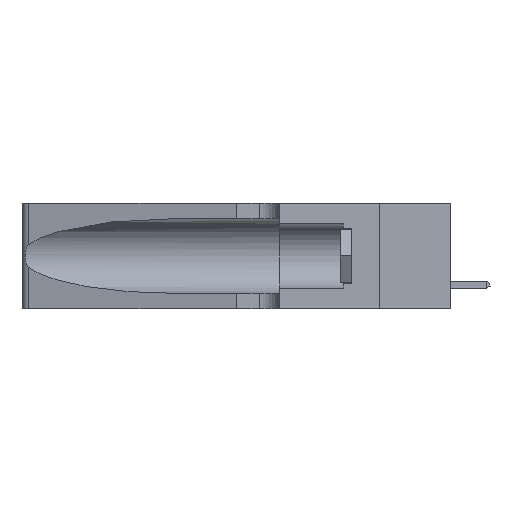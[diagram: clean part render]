
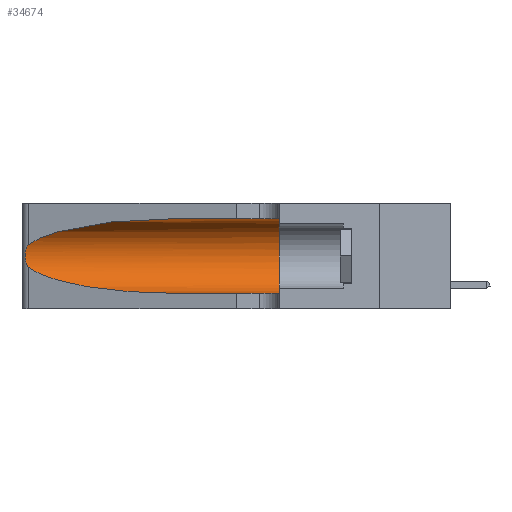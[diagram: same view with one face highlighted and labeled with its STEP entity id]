
A CAD part, left-side view. The second image highlights one B-rep face of the part: STEP entity #34674.
In plain terms, the highlighted cylindrical face has radius 3.308 mm (diameter 6.617 mm), a partial arc.
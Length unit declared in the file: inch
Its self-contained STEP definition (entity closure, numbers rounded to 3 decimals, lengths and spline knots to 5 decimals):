
#932 = EDGE_CURVE ( 'NONE', #12537, #33433, #32184, .T. ) ;
#1087 = VERTEX_POINT ( 'NONE', #41154 ) ;
#1741 = VECTOR ( 'NONE', #4543, 39.37008 ) ;
#1807 = CARTESIAN_POINT ( 'NONE',  ( 0.26018, 1.23835, 0.19895 ) ) ;
#2608 = DIRECTION ( 'NONE',  ( 0., 0., -1. ) ) ;
#2760 = CARTESIAN_POINT ( 'NONE',  ( 0.25487, 1.22718, 0.14631 ) ) ;
#2971 =( BOUNDED_CURVE ( )  B_SPLINE_CURVE ( 3, ( #9185, #18853, #9053, #19129 ),
 .UNSPECIFIED., .F., .T. ) 
 B_SPLINE_CURVE_WITH_KNOTS ( ( 4, 4 ),
 ( 1.5708, 2.84003 ),
 .UNSPECIFIED. ) 
 CURVE ( )  GEOMETRIC_REPRESENTATION_ITEM ( )  RATIONAL_B_SPLINE_CURVE ( ( 1., 0.87, 0.87, 1. ) ) 
 REPRESENTATION_ITEM ( '' )  );
#3777 = LINE ( 'NONE', #27806, #1741 ) ;
#3800 = CARTESIAN_POINT ( 'NONE',  ( 0.25487, 1.22718, 0.22369 ) ) ;
#3946 = FACE_OUTER_BOUND ( 'NONE', #23119, .T. ) ;
#4543 = DIRECTION ( 'NONE',  ( 0., -1., 0. ) ) ;
#4575 = DIRECTION ( 'NONE',  ( 0., 0., 1. ) ) ;
#5106 = CARTESIAN_POINT ( 'NONE',  ( 0.25789, 1.23486, 0.15765 ) ) ;
#8477 =( BOUNDED_CURVE ( )  B_SPLINE_CURVE ( 3, ( #30355, #37179, #30928, #40500 ),
 .UNSPECIFIED., .F., .F. ) 
 B_SPLINE_CURVE_WITH_KNOTS ( ( 4, 4 ),
 ( 3.44316, 4.71239 ),
 .UNSPECIFIED. ) 
 CURVE ( )  GEOMETRIC_REPRESENTATION_ITEM ( )  RATIONAL_B_SPLINE_CURVE ( ( 1., 0.87, 0.87, 1. ) ) 
 REPRESENTATION_ITEM ( '' )  );
#9053 = CARTESIAN_POINT ( 'NONE',  ( 0.2373, 1.15595, 0.28018 ) ) ;
#9185 = CARTESIAN_POINT ( 'NONE',  ( 0.1305, 0.72297, 0.31525 ) ) ;
#10622 = ORIENTED_EDGE ( 'NONE', *, *, #22939, .T. ) ;
#11042 = EDGE_CURVE ( 'NONE', #16119, #34407, #8477, .T. ) ;
#12537 = VERTEX_POINT ( 'NONE', #29027 ) ;
#13734 = ORIENTED_EDGE ( 'NONE', *, *, #40626, .F. ) ;
#14282 = ORIENTED_EDGE ( 'NONE', *, *, #932, .F. ) ;
#14436 = CARTESIAN_POINT ( 'NONE',  ( 0.25854, 1.2359, 0.20912 ) ) ;
#16119 = VERTEX_POINT ( 'NONE', #2760 ) ;
#18759 = EDGE_CURVE ( 'NONE', #23213, #16119, #30851, .T. ) ;
#18853 = CARTESIAN_POINT ( 'NONE',  ( 0.18966, 0.96281, 0.31525 ) ) ;
#19129 = CARTESIAN_POINT ( 'NONE',  ( 0.25487, 1.22718, 0.22369 ) ) ;
#21025 = CARTESIAN_POINT ( 'NONE',  ( 0.25856, 1.23593, 0.16098 ) ) ;
#21318 = CARTESIAN_POINT ( 'NONE',  ( 0.25555, 1.22993, 0.14849 ) ) ;
#21361 = CARTESIAN_POINT ( 'NONE',  ( 0.1305, 1.61858, 0.31525 ) ) ;
#22939 = EDGE_CURVE ( 'NONE', #34407, #33433, #3777, .T. ) ;
#23119 = EDGE_LOOP ( 'NONE', ( #31727, #27601, #33088, #10622, #14282, #13734 ) ) ;
#23213 = VERTEX_POINT ( 'NONE', #23945 ) ;
#23945 = CARTESIAN_POINT ( 'NONE',  ( 0.25487, 1.22718, 0.22369 ) ) ;
#24247 = DIRECTION ( 'NONE',  ( 0., 1., 0. ) ) ;
#24334 = CARTESIAN_POINT ( 'NONE',  ( 0.25639, 1.23186, 0.15144 ) ) ;
#26806 = VECTOR ( 'NONE', #28114, 39.37008 ) ;
#27601 = ORIENTED_EDGE ( 'NONE', *, *, #18759, .T. ) ;
#27806 = CARTESIAN_POINT ( 'NONE',  ( 0.1305, 1.61858, 0.05475 ) ) ;
#28114 = DIRECTION ( 'NONE',  ( 0., -1., 0. ) ) ;
#29027 = CARTESIAN_POINT ( 'NONE',  ( 0.1305, 0.35, 0.31525 ) ) ;
#30355 = CARTESIAN_POINT ( 'NONE',  ( 0.25487, 1.22718, 0.14631 ) ) ;
#30851 = B_SPLINE_CURVE_WITH_KNOTS ( 'NONE', 3,
 ( #3800, #40206, #37928, #40815, #14436, #1807, #37787, #40660, #34209, #21025, #5106, #24334, #21318, #31368 ),
 .UNSPECIFIED., .F., .F.,
 ( 4, 2, 2, 2, 2, 2, 4 ),
 ( 0., 0.00027, 0.00053, 0.00107, 0.0016, 0.00187, 0.00214 ),
 .UNSPECIFIED. ) ;
#30928 = CARTESIAN_POINT ( 'NONE',  ( 0.18966, 0.96281, 0.05475 ) ) ;
#31368 = CARTESIAN_POINT ( 'NONE',  ( 0.25487, 1.22718, 0.14631 ) ) ;
#31727 = ORIENTED_EDGE ( 'NONE', *, *, #36519, .T. ) ;
#32184 = CIRCLE ( 'NONE', #39343, 0.13025 ) ;
#32803 = CARTESIAN_POINT ( 'NONE',  ( 0.1305, 0.35, 0.05475 ) ) ;
#33088 = ORIENTED_EDGE ( 'NONE', *, *, #11042, .T. ) ;
#33433 = VERTEX_POINT ( 'NONE', #32803 ) ;
#34209 = CARTESIAN_POINT ( 'NONE',  ( 0.26017, 1.23833, 0.17102 ) ) ;
#34407 = VERTEX_POINT ( 'NONE', #35579 ) ;
#34674 = ADVANCED_FACE ( 'NONE', ( #3946 ), #37824, .F. ) ;
#35525 = LINE ( 'NONE', #21361, #26806 ) ;
#35579 = CARTESIAN_POINT ( 'NONE',  ( 0.1305, 0.72297, 0.05475 ) ) ;
#35925 = AXIS2_PLACEMENT_3D ( 'NONE', #37422, #40889, #2608 ) ;
#36519 = EDGE_CURVE ( 'NONE', #1087, #23213, #2971, .T. ) ;
#36799 = CARTESIAN_POINT ( 'NONE',  ( 0.1305, 0.35, 0.185 ) ) ;
#37179 = CARTESIAN_POINT ( 'NONE',  ( 0.2373, 1.15595, 0.08982 ) ) ;
#37422 = CARTESIAN_POINT ( 'NONE',  ( 0.1305, 1.61858, 0.185 ) ) ;
#37787 = CARTESIAN_POINT ( 'NONE',  ( 0.26075, 1.23896, 0.19203 ) ) ;
#37824 = CYLINDRICAL_SURFACE ( 'NONE', #35925, 0.13025 ) ;
#37928 = CARTESIAN_POINT ( 'NONE',  ( 0.25639, 1.23184, 0.21858 ) ) ;
#39343 = AXIS2_PLACEMENT_3D ( 'NONE', #36799, #24247, #4575 ) ;
#40206 = CARTESIAN_POINT ( 'NONE',  ( 0.25555, 1.22994, 0.2215 ) ) ;
#40500 = CARTESIAN_POINT ( 'NONE',  ( 0.1305, 0.72297, 0.05475 ) ) ;
#40626 = EDGE_CURVE ( 'NONE', #1087, #12537, #35525, .T. ) ;
#40660 = CARTESIAN_POINT ( 'NONE',  ( 0.26075, 1.23896, 0.178 ) ) ;
#40815 = CARTESIAN_POINT ( 'NONE',  ( 0.25787, 1.23484, 0.2124 ) ) ;
#40889 = DIRECTION ( 'NONE',  ( 0., -1., 0. ) ) ;
#41154 = CARTESIAN_POINT ( 'NONE',  ( 0.1305, 0.72297, 0.31525 ) ) ;
